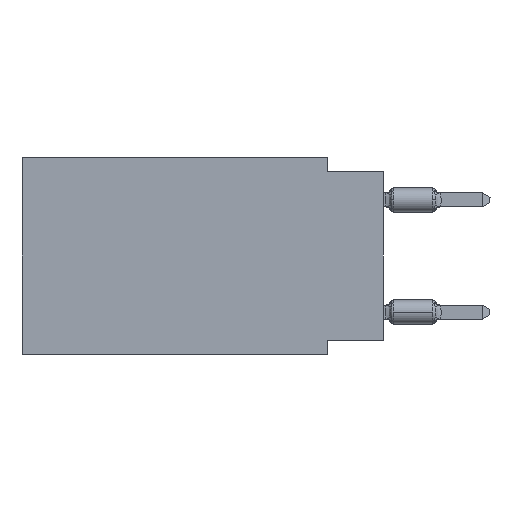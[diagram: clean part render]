
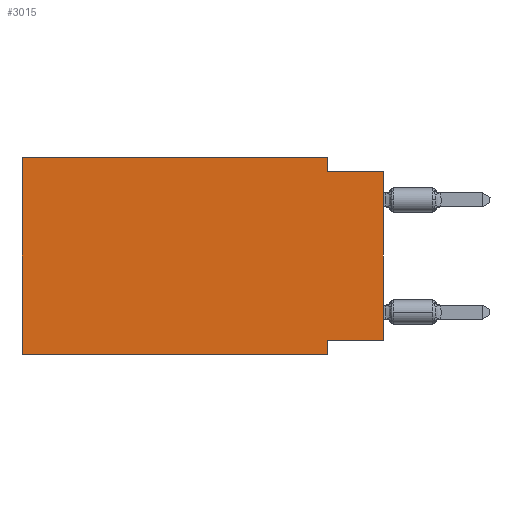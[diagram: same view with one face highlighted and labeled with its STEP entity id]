
A CAD part, left-side view. The second image highlights one B-rep face of the part: STEP entity #3015.
In plain terms, the highlighted planar face has unit normal (-1, 0, 0).
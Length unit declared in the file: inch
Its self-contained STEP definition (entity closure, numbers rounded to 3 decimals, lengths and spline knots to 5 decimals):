
#73 = LINE ( 'NONE', #1042, #19815 ) ;
#1042 = CARTESIAN_POINT ( 'NONE',  ( 0., 0.645, 0. ) ) ;
#3015 = ADVANCED_FACE ( 'NONE', ( #42885 ), #47677, .F. ) ;
#4045 = ORIENTED_EDGE ( 'NONE', *, *, #20638, .F. ) ;
#4787 = EDGE_CURVE ( 'NONE', #20983, #33484, #6264, .T. ) ;
#6264 = LINE ( 'NONE', #50520, #41127 ) ;
#8467 = CARTESIAN_POINT ( 'NONE',  ( 0., 0.1, -0.025 ) ) ;
#8582 = EDGE_CURVE ( 'NONE', #33484, #33290, #51344, .T. ) ;
#9746 = CARTESIAN_POINT ( 'NONE',  ( 0., 0.1, -0.325 ) ) ;
#11237 = VERTEX_POINT ( 'NONE', #27402 ) ;
#12313 = ORIENTED_EDGE ( 'NONE', *, *, #24710, .F. ) ;
#12974 = DIRECTION ( 'NONE',  ( 0., -1., 0. ) ) ;
#13848 = EDGE_LOOP ( 'NONE', ( #23980, #37536, #39974, #45386, #27726, #23810, #4045, #12313 ) ) ;
#14512 = CARTESIAN_POINT ( 'NONE',  ( 0., 0.1, 0. ) ) ;
#14793 = CARTESIAN_POINT ( 'NONE',  ( 0., 0.1, -0.35 ) ) ;
#18235 = LINE ( 'NONE', #30775, #29973 ) ;
#19815 = VECTOR ( 'NONE', #54524, 39.37008 ) ;
#20638 = EDGE_CURVE ( 'NONE', #33695, #31452, #34420, .T. ) ;
#20983 = VERTEX_POINT ( 'NONE', #14512 ) ;
#21717 = CARTESIAN_POINT ( 'NONE',  ( 0., 0., -0.025 ) ) ;
#23810 = ORIENTED_EDGE ( 'NONE', *, *, #27341, .T. ) ;
#23980 = ORIENTED_EDGE ( 'NONE', *, *, #30737, .T. ) ;
#24044 = CARTESIAN_POINT ( 'NONE',  ( 0., 0., -0.325 ) ) ;
#24331 = VECTOR ( 'NONE', #60253, 39.37008 ) ;
#24710 = EDGE_CURVE ( 'NONE', #42666, #33695, #49683, .T. ) ;
#27309 = LINE ( 'NONE', #56580, #48300 ) ;
#27341 = EDGE_CURVE ( 'NONE', #31612, #31452, #18235, .T. ) ;
#27402 = CARTESIAN_POINT ( 'NONE',  ( 0., 0.645, 0. ) ) ;
#27726 = ORIENTED_EDGE ( 'NONE', *, *, #61592, .F. ) ;
#29973 = VECTOR ( 'NONE', #50188, 39.37008 ) ;
#30737 = EDGE_CURVE ( 'NONE', #42666, #33290, #50743, .T. ) ;
#30775 = CARTESIAN_POINT ( 'NONE',  ( 0., 0.645, -0.35 ) ) ;
#31452 = VERTEX_POINT ( 'NONE', #14793 ) ;
#31612 = VERTEX_POINT ( 'NONE', #35476 ) ;
#32152 = VECTOR ( 'NONE', #54146, 39.37008 ) ;
#33151 = CARTESIAN_POINT ( 'NONE',  ( 0., 0., -0.025 ) ) ;
#33290 = VERTEX_POINT ( 'NONE', #33151 ) ;
#33484 = VERTEX_POINT ( 'NONE', #8467 ) ;
#33695 = VERTEX_POINT ( 'NONE', #9746 ) ;
#34420 = LINE ( 'NONE', #59552, #32152 ) ;
#35476 = CARTESIAN_POINT ( 'NONE',  ( 0., 0.645, -0.35 ) ) ;
#37536 = ORIENTED_EDGE ( 'NONE', *, *, #8582, .F. ) ;
#39974 = ORIENTED_EDGE ( 'NONE', *, *, #4787, .F. ) ;
#40217 = VECTOR ( 'NONE', #45934, 39.37008 ) ;
#41127 = VECTOR ( 'NONE', #45089, 39.37008 ) ;
#42278 = DIRECTION ( 'NONE',  ( 1., 0., 0. ) ) ;
#42666 = VERTEX_POINT ( 'NONE', #24044 ) ;
#42885 = FACE_OUTER_BOUND ( 'NONE', #13848, .T. ) ;
#44868 = EDGE_CURVE ( 'NONE', #11237, #20983, #27309, .T. ) ;
#45089 = DIRECTION ( 'NONE',  ( 0., 0., -1. ) ) ;
#45386 = ORIENTED_EDGE ( 'NONE', *, *, #44868, .F. ) ;
#45934 = DIRECTION ( 'NONE',  ( 0., 0., 1. ) ) ;
#47375 = DIRECTION ( 'NONE',  ( 0., 0., -1. ) ) ;
#47677 = PLANE ( 'NONE',  #62419 ) ;
#48300 = VECTOR ( 'NONE', #12974, 39.37008 ) ;
#49040 = DIRECTION ( 'NONE',  ( 0., 1., 0. ) ) ;
#49683 = LINE ( 'NONE', #59209, #54734 ) ;
#50188 = DIRECTION ( 'NONE',  ( 0., -1., 0. ) ) ;
#50520 = CARTESIAN_POINT ( 'NONE',  ( 0., 0.1, 0. ) ) ;
#50743 = LINE ( 'NONE', #60276, #40217 ) ;
#51344 = LINE ( 'NONE', #21717, #24331 ) ;
#54146 = DIRECTION ( 'NONE',  ( 0., 0., -1. ) ) ;
#54524 = DIRECTION ( 'NONE',  ( 0., 0., 1. ) ) ;
#54734 = VECTOR ( 'NONE', #49040, 39.37008 ) ;
#56580 = CARTESIAN_POINT ( 'NONE',  ( 0., 0.645, 0. ) ) ;
#57853 = CARTESIAN_POINT ( 'NONE',  ( 0., 0.645, 0. ) ) ;
#59209 = CARTESIAN_POINT ( 'NONE',  ( 0., 0., -0.325 ) ) ;
#59552 = CARTESIAN_POINT ( 'NONE',  ( 0., 0.1, -0.35 ) ) ;
#60253 = DIRECTION ( 'NONE',  ( 0., -1., 0. ) ) ;
#60276 = CARTESIAN_POINT ( 'NONE',  ( 0., 0., 0. ) ) ;
#61592 = EDGE_CURVE ( 'NONE', #31612, #11237, #73, .T. ) ;
#62419 = AXIS2_PLACEMENT_3D ( 'NONE', #57853, #42278, #47375 ) ;
